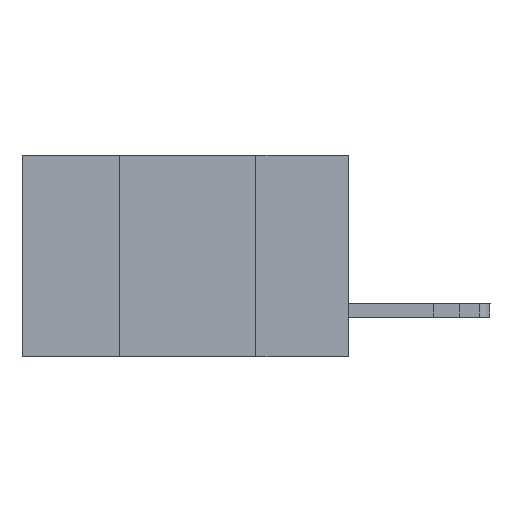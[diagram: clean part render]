
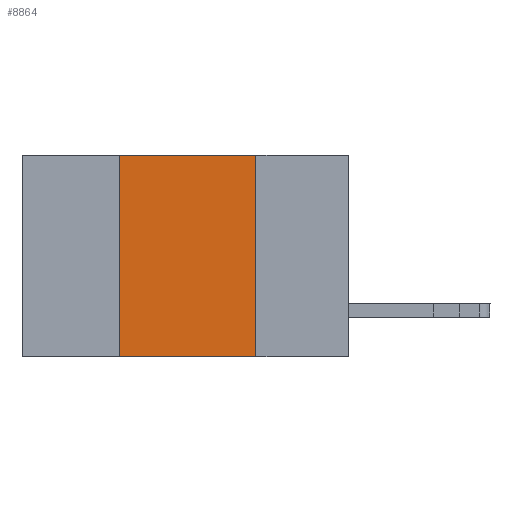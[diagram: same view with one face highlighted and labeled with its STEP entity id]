
A CAD part, left-side view. The second image highlights one B-rep face of the part: STEP entity #8864.
In plain terms, the highlighted planar face has unit normal (-1, 0, 0).
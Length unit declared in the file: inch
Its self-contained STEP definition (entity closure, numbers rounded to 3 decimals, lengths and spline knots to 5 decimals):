
#404 = VECTOR ( 'NONE', #5365, 39.37008 ) ;
#1608 = CARTESIAN_POINT ( 'NONE',  ( 0., 0.6, 0. ) ) ;
#1734 = VERTEX_POINT ( 'NONE', #3876 ) ;
#1967 = CARTESIAN_POINT ( 'NONE',  ( 0., 0.42, -0.37 ) ) ;
#2032 = CARTESIAN_POINT ( 'NONE',  ( 0., 0.42, 0. ) ) ;
#2109 = LINE ( 'NONE', #9960, #11562 ) ;
#2284 = DIRECTION ( 'NONE',  ( 0., -1., 0. ) ) ;
#2645 = DIRECTION ( 'NONE',  ( 0., 0., -1. ) ) ;
#3197 = EDGE_LOOP ( 'NONE', ( #11484, #6696, #3463, #11847 ) ) ;
#3463 = ORIENTED_EDGE ( 'NONE', *, *, #6501, .F. ) ;
#3876 = CARTESIAN_POINT ( 'NONE',  ( 0., 0.17, -0.37 ) ) ;
#3953 = VERTEX_POINT ( 'NONE', #5822 ) ;
#4141 = CARTESIAN_POINT ( 'NONE',  ( 0., 0.6, -0.37 ) ) ;
#4803 = AXIS2_PLACEMENT_3D ( 'NONE', #1608, #10499, #2645 ) ;
#4836 = EDGE_CURVE ( 'NONE', #8346, #3953, #2109, .T. ) ;
#5365 = DIRECTION ( 'NONE',  ( 0., 0., -1. ) ) ;
#5822 = CARTESIAN_POINT ( 'NONE',  ( 0., 0.17, 0. ) ) ;
#6351 = LINE ( 'NONE', #10137, #404 ) ;
#6501 = EDGE_CURVE ( 'NONE', #11195, #8346, #8038, .T. ) ;
#6657 = VECTOR ( 'NONE', #8990, 39.37008 ) ;
#6696 = ORIENTED_EDGE ( 'NONE', *, *, #4836, .F. ) ;
#6934 = EDGE_CURVE ( 'NONE', #11195, #1734, #11186, .T. ) ;
#6951 = CARTESIAN_POINT ( 'NONE',  ( 0., 0.42, -0.37 ) ) ;
#7474 = PLANE ( 'NONE',  #4803 ) ;
#7905 = DIRECTION ( 'NONE',  ( 0., -1., 0. ) ) ;
#8038 = LINE ( 'NONE', #6951, #6657 ) ;
#8346 = VERTEX_POINT ( 'NONE', #2032 ) ;
#8864 = ADVANCED_FACE ( 'NONE', ( #10379 ), #7474, .F. ) ;
#8910 = VECTOR ( 'NONE', #2284, 39.37008 ) ;
#8990 = DIRECTION ( 'NONE',  ( 0., 0., 1. ) ) ;
#9960 = CARTESIAN_POINT ( 'NONE',  ( 0., 0.6, 0. ) ) ;
#10137 = CARTESIAN_POINT ( 'NONE',  ( 0., 0.17, -0.37 ) ) ;
#10379 = FACE_OUTER_BOUND ( 'NONE', #3197, .T. ) ;
#10499 = DIRECTION ( 'NONE',  ( 1., 0., 0. ) ) ;
#11186 = LINE ( 'NONE', #4141, #8910 ) ;
#11195 = VERTEX_POINT ( 'NONE', #1967 ) ;
#11329 = EDGE_CURVE ( 'NONE', #3953, #1734, #6351, .T. ) ;
#11484 = ORIENTED_EDGE ( 'NONE', *, *, #11329, .F. ) ;
#11562 = VECTOR ( 'NONE', #7905, 39.37008 ) ;
#11847 = ORIENTED_EDGE ( 'NONE', *, *, #6934, .T. ) ;
